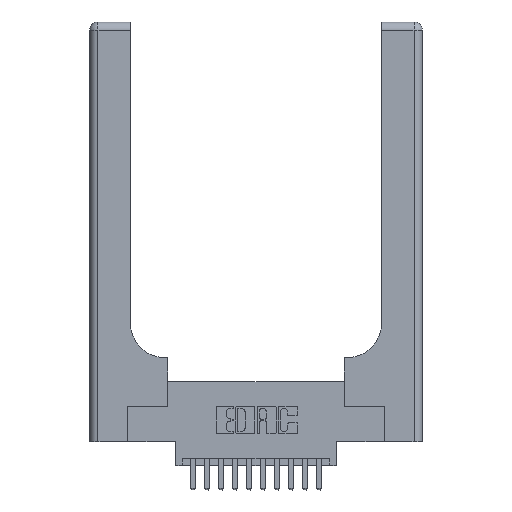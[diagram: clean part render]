
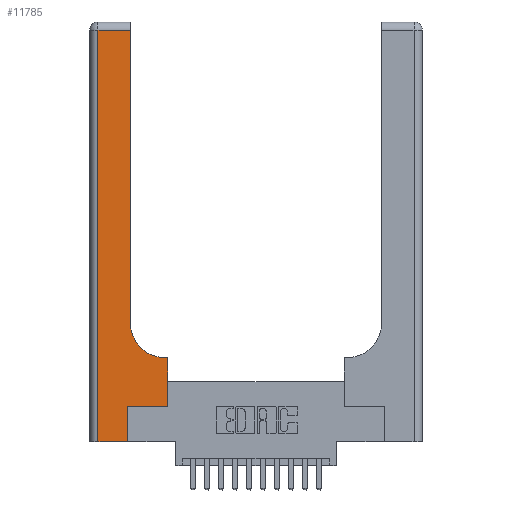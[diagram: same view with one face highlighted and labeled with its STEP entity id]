
A CAD part, top view. The second image highlights one B-rep face of the part: STEP entity #11785.
In plain terms, the highlighted planar face has unit normal (0, 0, 1).
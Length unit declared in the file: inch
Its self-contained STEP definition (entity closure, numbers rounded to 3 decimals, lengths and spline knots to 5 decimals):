
#157 = EDGE_CURVE ( 'NONE', #7686, #10844, #14156, .T. ) ;
#593 = LINE ( 'NONE', #8492, #3959 ) ;
#688 = CARTESIAN_POINT ( 'NONE',  ( 0., 0., 0.37 ) ) ;
#859 = DIRECTION ( 'NONE',  ( 0., 0., -1. ) ) ;
#879 = CARTESIAN_POINT ( 'NONE',  ( 0.2915, 2.94, 0.37 ) ) ;
#944 = CARTESIAN_POINT ( 'NONE',  ( 0.2915, 3., 0.37 ) ) ;
#1376 = VERTEX_POINT ( 'NONE', #13458 ) ;
#1767 = ORIENTED_EDGE ( 'NONE', *, *, #5949, .T. ) ;
#1921 = VERTEX_POINT ( 'NONE', #13305 ) ;
#2146 = DIRECTION ( 'NONE',  ( -1., 0., 0. ) ) ;
#2166 = CARTESIAN_POINT ( 'NONE',  ( 0.2915, 0.6, 0.37 ) ) ;
#2235 = VECTOR ( 'NONE', #11848, 39.37008 ) ;
#2539 = VECTOR ( 'NONE', #5313, 39.37008 ) ;
#2713 = ORIENTED_EDGE ( 'NONE', *, *, #6700, .T. ) ;
#2847 = AXIS2_PLACEMENT_3D ( 'NONE', #9082, #859, #10410 ) ;
#3149 = VECTOR ( 'NONE', #4984, 39.37008 ) ;
#3159 = EDGE_CURVE ( 'NONE', #15528, #12539, #9398, .T. ) ;
#3607 = LINE ( 'NONE', #14337, #3149 ) ;
#3718 = ORIENTED_EDGE ( 'NONE', *, *, #6795, .T. ) ;
#3763 = ORIENTED_EDGE ( 'NONE', *, *, #5579, .T. ) ;
#3921 = LINE ( 'NONE', #3962, #2539 ) ;
#3959 = VECTOR ( 'NONE', #12518, 39.37008 ) ;
#3962 = CARTESIAN_POINT ( 'NONE',  ( 0.06, 3., 0.37 ) ) ;
#4036 = VERTEX_POINT ( 'NONE', #9065 ) ;
#4134 = CARTESIAN_POINT ( 'NONE',  ( 0.5585, 0.6, 0.37 ) ) ;
#4402 = ORIENTED_EDGE ( 'NONE', *, *, #12835, .T. ) ;
#4723 = CIRCLE ( 'NONE', #9596, 0.25 ) ;
#4984 = DIRECTION ( 'NONE',  ( 0., 1., 0. ) ) ;
#5210 = VERTEX_POINT ( 'NONE', #6490 ) ;
#5313 = DIRECTION ( 'NONE',  ( 0., -1., 0. ) ) ;
#5348 = VECTOR ( 'NONE', #11588, 39.37008 ) ;
#5579 = EDGE_CURVE ( 'NONE', #13959, #7686, #13307, .T. ) ;
#5654 = EDGE_CURVE ( 'NONE', #5210, #1921, #12032, .T. ) ;
#5705 = CARTESIAN_POINT ( 'NONE',  ( 0.5415, 0.85, 0.37 ) ) ;
#5949 = EDGE_CURVE ( 'NONE', #10844, #1376, #4723, .T. ) ;
#6490 = CARTESIAN_POINT ( 'NONE',  ( 0.06, 0., 0.37 ) ) ;
#6700 = EDGE_CURVE ( 'NONE', #1921, #4036, #3607, .T. ) ;
#6795 = EDGE_CURVE ( 'NONE', #1376, #15528, #9899, .T. ) ;
#7064 = DIRECTION ( 'NONE',  ( 1., 0., 0. ) ) ;
#7459 = VECTOR ( 'NONE', #2146, 39.37008 ) ;
#7686 = VERTEX_POINT ( 'NONE', #4134 ) ;
#8111 = ORIENTED_EDGE ( 'NONE', *, *, #13895, .T. ) ;
#8492 = CARTESIAN_POINT ( 'NONE',  ( 0.269, 0.25, 0.37 ) ) ;
#8796 = CARTESIAN_POINT ( 'NONE',  ( 0.5585, 0.25, 0.37 ) ) ;
#9065 = CARTESIAN_POINT ( 'NONE',  ( 0.269, 0.25, 0.37 ) ) ;
#9082 = CARTESIAN_POINT ( 'NONE',  ( 0., 3., 0.37 ) ) ;
#9398 = LINE ( 'NONE', #16617, #16128 ) ;
#9596 = AXIS2_PLACEMENT_3D ( 'NONE', #5705, #15075, #7064 ) ;
#9899 = LINE ( 'NONE', #944, #2235 ) ;
#10410 = DIRECTION ( 'NONE',  ( -1., 0., 0. ) ) ;
#10486 = ORIENTED_EDGE ( 'NONE', *, *, #5654, .T. ) ;
#10686 = ORIENTED_EDGE ( 'NONE', *, *, #3159, .T. ) ;
#10725 = ORIENTED_EDGE ( 'NONE', *, *, #157, .T. ) ;
#10844 = VERTEX_POINT ( 'NONE', #14828 ) ;
#11197 = DIRECTION ( 'NONE',  ( -1., 0., 0. ) ) ;
#11588 = DIRECTION ( 'NONE',  ( 1., 0., 0. ) ) ;
#11785 = ADVANCED_FACE ( 'NONE', ( #11931 ), #17116, .F. ) ;
#11810 = EDGE_LOOP ( 'NONE', ( #3718, #10686, #8111, #10486, #2713, #4402, #3763, #10725, #1767 ) ) ;
#11848 = DIRECTION ( 'NONE',  ( 0., 1., 0. ) ) ;
#11931 = FACE_OUTER_BOUND ( 'NONE', #11810, .T. ) ;
#12032 = LINE ( 'NONE', #688, #5348 ) ;
#12082 = CARTESIAN_POINT ( 'NONE',  ( 0.5585, 0.25, 0.37 ) ) ;
#12518 = DIRECTION ( 'NONE',  ( 1., 0., 0. ) ) ;
#12539 = VERTEX_POINT ( 'NONE', #16002 ) ;
#12835 = EDGE_CURVE ( 'NONE', #4036, #13959, #593, .T. ) ;
#12850 = DIRECTION ( 'NONE',  ( 0., 1., 0. ) ) ;
#12889 = VECTOR ( 'NONE', #12850, 39.37008 ) ;
#13305 = CARTESIAN_POINT ( 'NONE',  ( 0.269, 0., 0.37 ) ) ;
#13307 = LINE ( 'NONE', #8796, #12889 ) ;
#13458 = CARTESIAN_POINT ( 'NONE',  ( 0.2915, 0.85, 0.37 ) ) ;
#13895 = EDGE_CURVE ( 'NONE', #12539, #5210, #3921, .T. ) ;
#13959 = VERTEX_POINT ( 'NONE', #12082 ) ;
#14156 = LINE ( 'NONE', #2166, #7459 ) ;
#14337 = CARTESIAN_POINT ( 'NONE',  ( 0.269, 0., 0.37 ) ) ;
#14828 = CARTESIAN_POINT ( 'NONE',  ( 0.5415, 0.6, 0.37 ) ) ;
#15075 = DIRECTION ( 'NONE',  ( 0., 0., -1. ) ) ;
#15528 = VERTEX_POINT ( 'NONE', #879 ) ;
#16002 = CARTESIAN_POINT ( 'NONE',  ( 0.06, 2.94, 0.37 ) ) ;
#16128 = VECTOR ( 'NONE', #11197, 39.37008 ) ;
#16617 = CARTESIAN_POINT ( 'NONE',  ( 0., 2.94, 0.37 ) ) ;
#17116 = PLANE ( 'NONE',  #2847 ) ;
